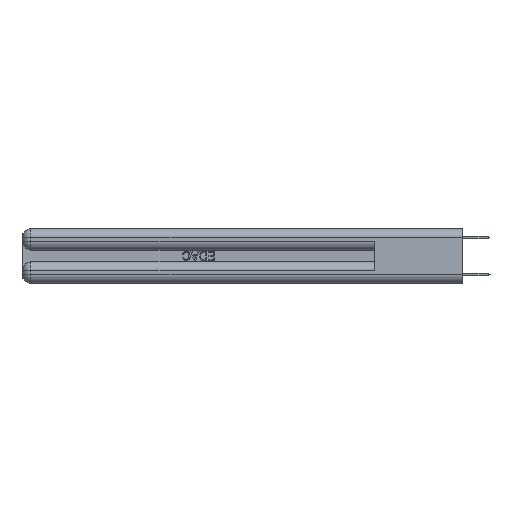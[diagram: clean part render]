
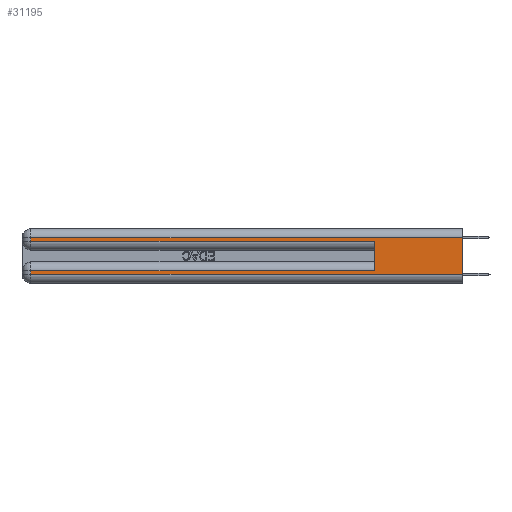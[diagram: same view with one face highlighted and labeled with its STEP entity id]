
A CAD part, left-side view. The second image highlights one B-rep face of the part: STEP entity #31195.
In plain terms, the highlighted planar face has unit normal (-1, 0, 0).
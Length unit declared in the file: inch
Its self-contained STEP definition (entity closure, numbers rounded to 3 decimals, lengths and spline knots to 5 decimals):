
#150 = ORIENTED_EDGE ( 'NONE', *, *, #30683, .T. ) ;
#476 = CARTESIAN_POINT ( 'NONE',  ( 0., 0., 0.085 ) ) ;
#943 = VECTOR ( 'NONE', #2454, 39.37008 ) ;
#2012 = VERTEX_POINT ( 'NONE', #16457 ) ;
#2169 = ORIENTED_EDGE ( 'NONE', *, *, #23324, .T. ) ;
#2175 = ORIENTED_EDGE ( 'NONE', *, *, #6662, .T. ) ;
#2454 = DIRECTION ( 'NONE',  ( 0., 1., 0. ) ) ;
#3576 = VECTOR ( 'NONE', #15276, 39.37008 ) ;
#3724 = LINE ( 'NONE', #16082, #21816 ) ;
#4982 = CARTESIAN_POINT ( 'NONE',  ( 0., 2.94, 0.285 ) ) ;
#5371 = CARTESIAN_POINT ( 'NONE',  ( 0., 0., 0.37 ) ) ;
#6325 = CARTESIAN_POINT ( 'NONE',  ( 0., 0., 0.285 ) ) ;
#6662 = EDGE_CURVE ( 'NONE', #28345, #13063, #9567, .T. ) ;
#7107 = CARTESIAN_POINT ( 'NONE',  ( 0., 0.6, 0.085 ) ) ;
#7280 = EDGE_LOOP ( 'NONE', ( #25169, #20962, #2175, #2169, #16655, #150, #16077, #15110 ) ) ;
#7656 = LINE ( 'NONE', #19694, #943 ) ;
#7719 = VERTEX_POINT ( 'NONE', #14315 ) ;
#8112 = CARTESIAN_POINT ( 'NONE',  ( 0., 0., 0.06 ) ) ;
#9258 = CARTESIAN_POINT ( 'NONE',  ( 0., 0.6, 0.285 ) ) ;
#9420 = VECTOR ( 'NONE', #17227, 39.37008 ) ;
#9567 = LINE ( 'NONE', #24536, #9420 ) ;
#9752 = VERTEX_POINT ( 'NONE', #7107 ) ;
#10396 = DIRECTION ( 'NONE',  ( 0., 1., 0. ) ) ;
#10551 = LINE ( 'NONE', #476, #26291 ) ;
#10784 = LINE ( 'NONE', #20716, #27946 ) ;
#12423 = VERTEX_POINT ( 'NONE', #9258 ) ;
#12664 = DIRECTION ( 'NONE',  ( 0., -1., 0. ) ) ;
#13063 = VERTEX_POINT ( 'NONE', #4982 ) ;
#13686 = EDGE_CURVE ( 'NONE', #16223, #2012, #10784, .T. ) ;
#14005 = EDGE_CURVE ( 'NONE', #2012, #21952, #27469, .T. ) ;
#14315 = CARTESIAN_POINT ( 'NONE',  ( 0., 0., 0.31 ) ) ;
#15110 = ORIENTED_EDGE ( 'NONE', *, *, #14005, .T. ) ;
#15276 = DIRECTION ( 'NONE',  ( 0., 0., -1. ) ) ;
#15756 = CARTESIAN_POINT ( 'NONE',  ( 0., 0., 0.06 ) ) ;
#16051 = FACE_OUTER_BOUND ( 'NONE', #7280, .T. ) ;
#16077 = ORIENTED_EDGE ( 'NONE', *, *, #13686, .T. ) ;
#16082 = CARTESIAN_POINT ( 'NONE',  ( 0., 0.6, 0.145 ) ) ;
#16223 = VERTEX_POINT ( 'NONE', #22926 ) ;
#16258 = EDGE_CURVE ( 'NONE', #7719, #21952, #25525, .T. ) ;
#16457 = CARTESIAN_POINT ( 'NONE',  ( 0., 2.94, 0.06 ) ) ;
#16655 = ORIENTED_EDGE ( 'NONE', *, *, #23362, .F. ) ;
#17227 = DIRECTION ( 'NONE',  ( 0., 0., -1. ) ) ;
#17997 = DIRECTION ( 'NONE',  ( 1., 0., 0. ) ) ;
#19018 = EDGE_CURVE ( 'NONE', #7719, #28345, #7656, .T. ) ;
#19694 = CARTESIAN_POINT ( 'NONE',  ( 0., 0., 0.31 ) ) ;
#20716 = CARTESIAN_POINT ( 'NONE',  ( 0., 2.94, 0.37 ) ) ;
#20962 = ORIENTED_EDGE ( 'NONE', *, *, #19018, .T. ) ;
#21816 = VECTOR ( 'NONE', #25992, 39.37008 ) ;
#21952 = VERTEX_POINT ( 'NONE', #15756 ) ;
#22926 = CARTESIAN_POINT ( 'NONE',  ( 0., 2.94, 0.085 ) ) ;
#23324 = EDGE_CURVE ( 'NONE', #13063, #12423, #30871, .T. ) ;
#23362 = EDGE_CURVE ( 'NONE', #9752, #12423, #3724, .T. ) ;
#23394 = DIRECTION ( 'NONE',  ( 0., -1., 0. ) ) ;
#24536 = CARTESIAN_POINT ( 'NONE',  ( 0., 2.94, 0.37 ) ) ;
#24942 = VECTOR ( 'NONE', #23394, 39.37008 ) ;
#25169 = ORIENTED_EDGE ( 'NONE', *, *, #16258, .F. ) ;
#25484 = PLANE ( 'NONE',  #27888 ) ;
#25525 = LINE ( 'NONE', #5371, #3576 ) ;
#25992 = DIRECTION ( 'NONE',  ( 0., 0., 1. ) ) ;
#26250 = CARTESIAN_POINT ( 'NONE',  ( 0., 2.94, 0.31 ) ) ;
#26291 = VECTOR ( 'NONE', #10396, 39.37008 ) ;
#26404 = VECTOR ( 'NONE', #12664, 39.37008 ) ;
#27469 = LINE ( 'NONE', #8112, #26404 ) ;
#27888 = AXIS2_PLACEMENT_3D ( 'NONE', #30364, #17997, #27917 ) ;
#27917 = DIRECTION ( 'NONE',  ( 0., 0., -1. ) ) ;
#27946 = VECTOR ( 'NONE', #30477, 39.37008 ) ;
#28345 = VERTEX_POINT ( 'NONE', #26250 ) ;
#30364 = CARTESIAN_POINT ( 'NONE',  ( 0., 0., 0.37 ) ) ;
#30477 = DIRECTION ( 'NONE',  ( 0., 0., -1. ) ) ;
#30683 = EDGE_CURVE ( 'NONE', #9752, #16223, #10551, .T. ) ;
#30871 = LINE ( 'NONE', #6325, #24942 ) ;
#31195 = ADVANCED_FACE ( 'NONE', ( #16051 ), #25484, .F. ) ;
